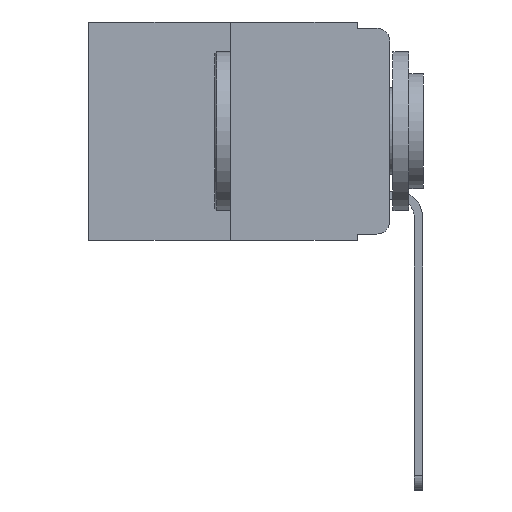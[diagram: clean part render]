
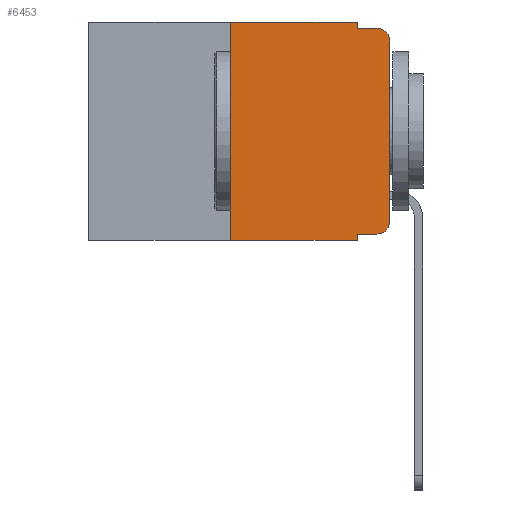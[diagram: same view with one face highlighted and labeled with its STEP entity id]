
A CAD part, left-side view. The second image highlights one B-rep face of the part: STEP entity #6453.
In plain terms, the highlighted planar face has unit normal (-1, 0, 0).
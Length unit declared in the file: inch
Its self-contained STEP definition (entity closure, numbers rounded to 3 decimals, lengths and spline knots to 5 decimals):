
#94 = ORIENTED_EDGE ( 'NONE', *, *, #11963, .T. ) ;
#582 = CARTESIAN_POINT ( 'NONE',  ( 0., 0.25, -0.343 ) ) ;
#918 = AXIS2_PLACEMENT_3D ( 'NONE', #14559, #4217, #16235 ) ;
#2139 = VERTEX_POINT ( 'NONE', #16213 ) ;
#2401 = AXIS2_PLACEMENT_3D ( 'NONE', #9662, #21333, #11382 ) ;
#2910 = VERTEX_POINT ( 'NONE', #11584 ) ;
#2940 = ORIENTED_EDGE ( 'NONE', *, *, #14693, .F. ) ;
#3134 = CARTESIAN_POINT ( 'NONE',  ( 0., 0.02, -0.333 ) ) ;
#3965 = VERTEX_POINT ( 'NONE', #11702 ) ;
#4150 = ORIENTED_EDGE ( 'NONE', *, *, #7707, .T. ) ;
#4217 = DIRECTION ( 'NONE',  ( -1., 0., 0. ) ) ;
#4546 = LINE ( 'NONE', #8875, #21449 ) ;
#4808 = EDGE_CURVE ( 'NONE', #15064, #22403, #10473, .T. ) ;
#5193 = EDGE_LOOP ( 'NONE', ( #14697, #10701, #19616, #6670, #2940, #12316, #4150, #22117, #9372, #94 ) ) ;
#5223 = DIRECTION ( 'NONE',  ( 0., 0., 1. ) ) ;
#5573 = EDGE_CURVE ( 'NONE', #19730, #2910, #12039, .T. ) ;
#5862 = VECTOR ( 'NONE', #15388, 39.37008 ) ;
#5885 = VECTOR ( 'NONE', #9193, 39.37008 ) ;
#6013 = EDGE_CURVE ( 'NONE', #22403, #6491, #14675, .T. ) ;
#6453 = ADVANCED_FACE ( 'NONE', ( #19573 ), #18094, .F. ) ;
#6491 = VERTEX_POINT ( 'NONE', #19722 ) ;
#6670 = ORIENTED_EDGE ( 'NONE', *, *, #8322, .F. ) ;
#6891 = CARTESIAN_POINT ( 'NONE',  ( 0., 0.02, -0.03 ) ) ;
#6932 = LINE ( 'NONE', #19250, #5885 ) ;
#7142 = EDGE_CURVE ( 'NONE', #3965, #6491, #11958, .T. ) ;
#7420 = VECTOR ( 'NONE', #9476, 39.37008 ) ;
#7494 = VECTOR ( 'NONE', #5223, 39.37008 ) ;
#7700 = LINE ( 'NONE', #21028, #15643 ) ;
#7707 = EDGE_CURVE ( 'NONE', #19730, #18474, #6932, .T. ) ;
#7791 = CARTESIAN_POINT ( 'NONE',  ( 0., 0., 0. ) ) ;
#8322 = EDGE_CURVE ( 'NONE', #13004, #3965, #14930, .T. ) ;
#8645 = DIRECTION ( 'NONE',  ( 0., 0., -1. ) ) ;
#8875 = CARTESIAN_POINT ( 'NONE',  ( 0., 0.051, 0. ) ) ;
#9193 = DIRECTION ( 'NONE',  ( 0., -1., 0. ) ) ;
#9208 = LINE ( 'NONE', #10602, #17656 ) ;
#9372 = ORIENTED_EDGE ( 'NONE', *, *, #12740, .T. ) ;
#9476 = DIRECTION ( 'NONE',  ( 0., -1., 0. ) ) ;
#9662 = CARTESIAN_POINT ( 'NONE',  ( 0., 0.473, 0. ) ) ;
#9925 = VECTOR ( 'NONE', #17890, 39.37008 ) ;
#10296 = CARTESIAN_POINT ( 'NONE',  ( 0., 0.051, 0. ) ) ;
#10473 = LINE ( 'NONE', #7791, #9925 ) ;
#10579 = DIRECTION ( 'NONE',  ( 0., 0., -1. ) ) ;
#10580 = CIRCLE ( 'NONE', #918, 0.02 ) ;
#10602 = CARTESIAN_POINT ( 'NONE',  ( 0., 0.051, -0.333 ) ) ;
#10701 = ORIENTED_EDGE ( 'NONE', *, *, #6013, .T. ) ;
#11382 = DIRECTION ( 'NONE',  ( 0., 0., -1. ) ) ;
#11411 = CARTESIAN_POINT ( 'NONE',  ( 0., 0.051, 0. ) ) ;
#11584 = CARTESIAN_POINT ( 'NONE',  ( 0., 0.25, 0. ) ) ;
#11702 = CARTESIAN_POINT ( 'NONE',  ( 0., 0.051, -0.01 ) ) ;
#11958 = LINE ( 'NONE', #12808, #7420 ) ;
#11963 = EDGE_CURVE ( 'NONE', #13705, #15064, #10580, .T. ) ;
#12039 = LINE ( 'NONE', #18726, #7494 ) ;
#12316 = ORIENTED_EDGE ( 'NONE', *, *, #5573, .F. ) ;
#12339 = DIRECTION ( 'NONE',  ( 0., -1., 0. ) ) ;
#12740 = EDGE_CURVE ( 'NONE', #2139, #13705, #9208, .T. ) ;
#12808 = CARTESIAN_POINT ( 'NONE',  ( 0., 0.051, -0.01 ) ) ;
#13004 = VERTEX_POINT ( 'NONE', #11411 ) ;
#13213 = EDGE_CURVE ( 'NONE', #2139, #18474, #4546, .T. ) ;
#13542 = CARTESIAN_POINT ( 'NONE',  ( 0., 0., -0.313 ) ) ;
#13653 = CARTESIAN_POINT ( 'NONE',  ( 0., 0.051, -0.343 ) ) ;
#13705 = VERTEX_POINT ( 'NONE', #3134 ) ;
#14507 = DIRECTION ( 'NONE',  ( 0., -1., 0. ) ) ;
#14559 = CARTESIAN_POINT ( 'NONE',  ( 0., 0.02, -0.313 ) ) ;
#14675 = CIRCLE ( 'NONE', #15024, 0.02 ) ;
#14693 = EDGE_CURVE ( 'NONE', #2910, #13004, #7700, .T. ) ;
#14697 = ORIENTED_EDGE ( 'NONE', *, *, #4808, .T. ) ;
#14930 = LINE ( 'NONE', #10296, #5862 ) ;
#15024 = AXIS2_PLACEMENT_3D ( 'NONE', #6891, #18730, #8645 ) ;
#15064 = VERTEX_POINT ( 'NONE', #13542 ) ;
#15388 = DIRECTION ( 'NONE',  ( 0., 0., -1. ) ) ;
#15643 = VECTOR ( 'NONE', #14507, 39.37008 ) ;
#16213 = CARTESIAN_POINT ( 'NONE',  ( 0., 0.051, -0.333 ) ) ;
#16235 = DIRECTION ( 'NONE',  ( 0., 0., -1. ) ) ;
#17656 = VECTOR ( 'NONE', #12339, 39.37008 ) ;
#17890 = DIRECTION ( 'NONE',  ( 0., 0., 1. ) ) ;
#17907 = CARTESIAN_POINT ( 'NONE',  ( 0., 0., -0.03 ) ) ;
#18094 = PLANE ( 'NONE',  #2401 ) ;
#18474 = VERTEX_POINT ( 'NONE', #13653 ) ;
#18726 = CARTESIAN_POINT ( 'NONE',  ( 0., 0.25, 0. ) ) ;
#18730 = DIRECTION ( 'NONE',  ( -1., 0., 0. ) ) ;
#19250 = CARTESIAN_POINT ( 'NONE',  ( 0., 0.473, -0.343 ) ) ;
#19573 = FACE_OUTER_BOUND ( 'NONE', #5193, .T. ) ;
#19616 = ORIENTED_EDGE ( 'NONE', *, *, #7142, .F. ) ;
#19722 = CARTESIAN_POINT ( 'NONE',  ( 0., 0.02, -0.01 ) ) ;
#19730 = VERTEX_POINT ( 'NONE', #582 ) ;
#21028 = CARTESIAN_POINT ( 'NONE',  ( 0., 0.473, 0. ) ) ;
#21333 = DIRECTION ( 'NONE',  ( 1., 0., 0. ) ) ;
#21449 = VECTOR ( 'NONE', #10579, 39.37008 ) ;
#22117 = ORIENTED_EDGE ( 'NONE', *, *, #13213, .F. ) ;
#22403 = VERTEX_POINT ( 'NONE', #17907 ) ;
